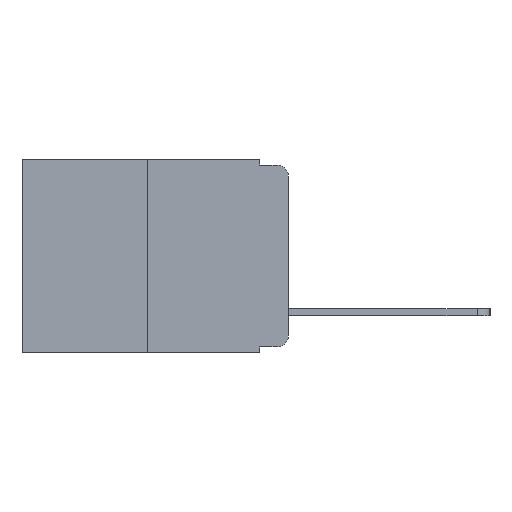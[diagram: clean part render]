
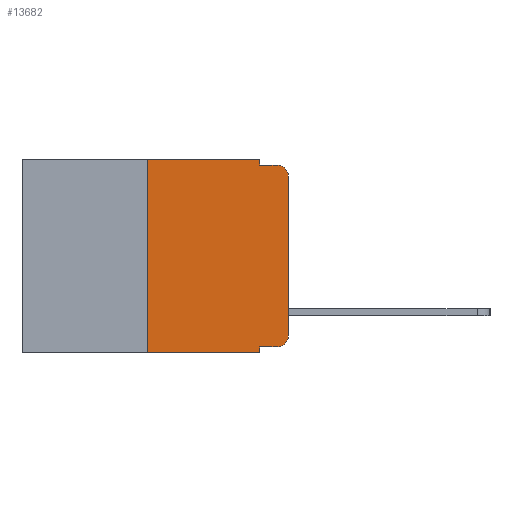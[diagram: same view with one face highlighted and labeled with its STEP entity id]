
A CAD part, left-side view. The second image highlights one B-rep face of the part: STEP entity #13682.
In plain terms, the highlighted planar face has unit normal (-1, 0, 0).
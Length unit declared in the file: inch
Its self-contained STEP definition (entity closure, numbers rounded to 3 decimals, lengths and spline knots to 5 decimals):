
#1251 = CARTESIAN_POINT ( 'NONE',  ( 0., 0.051, 0. ) ) ;
#1319 = FACE_OUTER_BOUND ( 'NONE', #19493, .T. ) ;
#1432 = VERTEX_POINT ( 'NONE', #1777 ) ;
#1468 = CARTESIAN_POINT ( 'NONE',  ( 0., 0., -0.03 ) ) ;
#1777 = CARTESIAN_POINT ( 'NONE',  ( 0., 0.25, 0. ) ) ;
#2758 = DIRECTION ( 'NONE',  ( 0., 0., -1. ) ) ;
#2778 = CARTESIAN_POINT ( 'NONE',  ( 0., 0.25, 0. ) ) ;
#2876 = CARTESIAN_POINT ( 'NONE',  ( 0., 0.473, -0.343 ) ) ;
#3023 = LINE ( 'NONE', #2876, #12782 ) ;
#3538 = VECTOR ( 'NONE', #20798, 39.37008 ) ;
#3694 = ORIENTED_EDGE ( 'NONE', *, *, #9934, .T. ) ;
#3881 = VERTEX_POINT ( 'NONE', #23335 ) ;
#3887 = VERTEX_POINT ( 'NONE', #15956 ) ;
#4741 = DIRECTION ( 'NONE',  ( 0., 0., 1. ) ) ;
#4764 = DIRECTION ( 'NONE',  ( 0., 0., 1. ) ) ;
#4787 = VECTOR ( 'NONE', #6183, 39.37008 ) ;
#4848 = DIRECTION ( 'NONE',  ( 0., -1., 0. ) ) ;
#4934 = VECTOR ( 'NONE', #19130, 39.37008 ) ;
#5124 = CARTESIAN_POINT ( 'NONE',  ( 0., 0.051, -0.01 ) ) ;
#5218 = ORIENTED_EDGE ( 'NONE', *, *, #17625, .T. ) ;
#5391 = AXIS2_PLACEMENT_3D ( 'NONE', #11691, #24732, #13615 ) ;
#5415 = LINE ( 'NONE', #21931, #20675 ) ;
#5801 = ORIENTED_EDGE ( 'NONE', *, *, #16342, .F. ) ;
#5914 = VECTOR ( 'NONE', #2758, 39.37008 ) ;
#6048 = VERTEX_POINT ( 'NONE', #7090 ) ;
#6183 = DIRECTION ( 'NONE',  ( 0., -1., 0. ) ) ;
#7056 = ORIENTED_EDGE ( 'NONE', *, *, #23370, .F. ) ;
#7090 = CARTESIAN_POINT ( 'NONE',  ( 0., 0.051, -0.333 ) ) ;
#7314 = VERTEX_POINT ( 'NONE', #20738 ) ;
#7653 = CARTESIAN_POINT ( 'NONE',  ( 0., 0.473, 0. ) ) ;
#8145 = PLANE ( 'NONE',  #13479 ) ;
#8257 = ORIENTED_EDGE ( 'NONE', *, *, #11229, .T. ) ;
#8305 = CIRCLE ( 'NONE', #19255, 0.02 ) ;
#8649 = LINE ( 'NONE', #2778, #13213 ) ;
#8957 = CARTESIAN_POINT ( 'NONE',  ( 0., 0.051, 0. ) ) ;
#9793 = VERTEX_POINT ( 'NONE', #1468 ) ;
#9878 = CIRCLE ( 'NONE', #5391, 0.02 ) ;
#9934 = EDGE_CURVE ( 'NONE', #10788, #7314, #8305, .T. ) ;
#10130 = DIRECTION ( 'NONE',  ( 0., 0., -1. ) ) ;
#10131 = LINE ( 'NONE', #7653, #4934 ) ;
#10305 = VERTEX_POINT ( 'NONE', #5124 ) ;
#10534 = CARTESIAN_POINT ( 'NONE',  ( 0., 0.051, 0. ) ) ;
#10605 = LINE ( 'NONE', #19599, #4787 ) ;
#10788 = VERTEX_POINT ( 'NONE', #20180 ) ;
#11016 = ORIENTED_EDGE ( 'NONE', *, *, #15086, .F. ) ;
#11123 = LINE ( 'NONE', #10534, #5914 ) ;
#11229 = EDGE_CURVE ( 'NONE', #6048, #10788, #10605, .T. ) ;
#11691 = CARTESIAN_POINT ( 'NONE',  ( 0., 0.02, -0.03 ) ) ;
#11716 = DIRECTION ( 'NONE',  ( -1., 0., 0. ) ) ;
#12120 = VERTEX_POINT ( 'NONE', #8957 ) ;
#12235 = ORIENTED_EDGE ( 'NONE', *, *, #13806, .F. ) ;
#12540 = EDGE_CURVE ( 'NONE', #6048, #3887, #11123, .T. ) ;
#12782 = VECTOR ( 'NONE', #4848, 39.37008 ) ;
#13213 = VECTOR ( 'NONE', #4741, 39.37008 ) ;
#13479 = AXIS2_PLACEMENT_3D ( 'NONE', #19604, #21438, #10130 ) ;
#13615 = DIRECTION ( 'NONE',  ( 0., 0., -1. ) ) ;
#13682 = ADVANCED_FACE ( 'NONE', ( #1319 ), #8145, .F. ) ;
#13806 = EDGE_CURVE ( 'NONE', #3881, #1432, #8649, .T. ) ;
#14474 = LINE ( 'NONE', #18968, #3538 ) ;
#15086 = EDGE_CURVE ( 'NONE', #12120, #10305, #23644, .T. ) ;
#15956 = CARTESIAN_POINT ( 'NONE',  ( 0., 0.051, -0.343 ) ) ;
#16239 = CARTESIAN_POINT ( 'NONE',  ( 0., 0.02, -0.01 ) ) ;
#16342 = EDGE_CURVE ( 'NONE', #10305, #24378, #14474, .T. ) ;
#17625 = EDGE_CURVE ( 'NONE', #9793, #24378, #9878, .T. ) ;
#18667 = DIRECTION ( 'NONE',  ( 0., 0., -1. ) ) ;
#18776 = VECTOR ( 'NONE', #18667, 39.37008 ) ;
#18968 = CARTESIAN_POINT ( 'NONE',  ( 0., 0.051, -0.01 ) ) ;
#19130 = DIRECTION ( 'NONE',  ( 0., -1., 0. ) ) ;
#19255 = AXIS2_PLACEMENT_3D ( 'NONE', #22930, #11716, #24753 ) ;
#19320 = ORIENTED_EDGE ( 'NONE', *, *, #21329, .T. ) ;
#19493 = EDGE_LOOP ( 'NONE', ( #19320, #5218, #5801, #11016, #7056, #12235, #22208, #22776, #8257, #3694 ) ) ;
#19599 = CARTESIAN_POINT ( 'NONE',  ( 0., 0.051, -0.333 ) ) ;
#19604 = CARTESIAN_POINT ( 'NONE',  ( 0., 0.473, 0. ) ) ;
#19956 = EDGE_CURVE ( 'NONE', #3881, #3887, #3023, .T. ) ;
#20180 = CARTESIAN_POINT ( 'NONE',  ( 0., 0.02, -0.333 ) ) ;
#20675 = VECTOR ( 'NONE', #4764, 39.37008 ) ;
#20738 = CARTESIAN_POINT ( 'NONE',  ( 0., 0., -0.313 ) ) ;
#20798 = DIRECTION ( 'NONE',  ( 0., -1., 0. ) ) ;
#21329 = EDGE_CURVE ( 'NONE', #7314, #9793, #5415, .T. ) ;
#21438 = DIRECTION ( 'NONE',  ( 1., 0., 0. ) ) ;
#21931 = CARTESIAN_POINT ( 'NONE',  ( 0., 0., 0. ) ) ;
#22208 = ORIENTED_EDGE ( 'NONE', *, *, #19956, .T. ) ;
#22776 = ORIENTED_EDGE ( 'NONE', *, *, #12540, .F. ) ;
#22930 = CARTESIAN_POINT ( 'NONE',  ( 0., 0.02, -0.313 ) ) ;
#23335 = CARTESIAN_POINT ( 'NONE',  ( 0., 0.25, -0.343 ) ) ;
#23370 = EDGE_CURVE ( 'NONE', #1432, #12120, #10131, .T. ) ;
#23644 = LINE ( 'NONE', #1251, #18776 ) ;
#24378 = VERTEX_POINT ( 'NONE', #16239 ) ;
#24732 = DIRECTION ( 'NONE',  ( -1., 0., 0. ) ) ;
#24753 = DIRECTION ( 'NONE',  ( 0., 0., -1. ) ) ;
